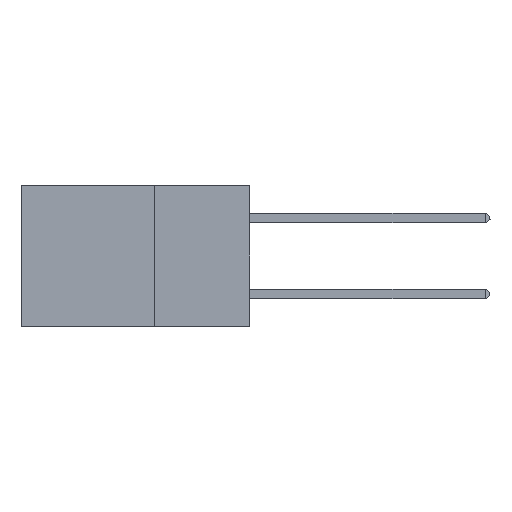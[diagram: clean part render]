
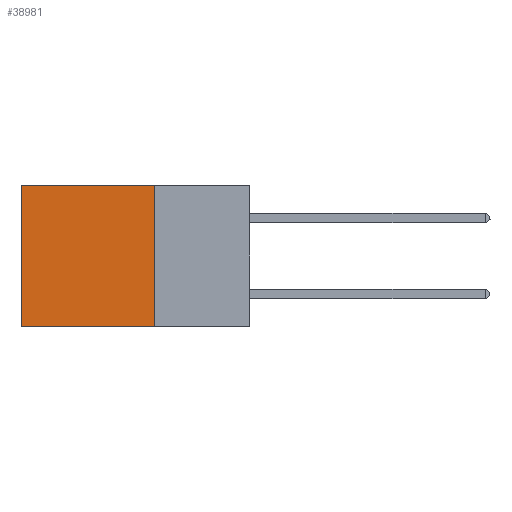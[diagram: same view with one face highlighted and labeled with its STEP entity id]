
A CAD part, left-side view. The second image highlights one B-rep face of the part: STEP entity #38981.
In plain terms, the highlighted planar face has unit normal (-1, 0, 0).
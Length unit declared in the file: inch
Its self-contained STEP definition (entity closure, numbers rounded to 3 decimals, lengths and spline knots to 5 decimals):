
#586 = CARTESIAN_POINT ( 'NONE',  ( 0.2875, 0.6, -0.37 ) ) ;
#1732 = ORIENTED_EDGE ( 'NONE', *, *, #22450, .T. ) ;
#2287 = DIRECTION ( 'NONE',  ( 0., 0., -1. ) ) ;
#5880 = ORIENTED_EDGE ( 'NONE', *, *, #6147, .F. ) ;
#6147 = EDGE_CURVE ( 'NONE', #39737, #12681, #35643, .T. ) ;
#6818 = CARTESIAN_POINT ( 'NONE',  ( 0.2875, 0.25, 0. ) ) ;
#7216 = DIRECTION ( 'NONE',  ( 0., 1., 0. ) ) ;
#8172 = LINE ( 'NONE', #26784, #22308 ) ;
#8890 = CARTESIAN_POINT ( 'NONE',  ( 0.2875, 0.6, 0. ) ) ;
#9580 = EDGE_CURVE ( 'NONE', #12681, #25426, #8172, .T. ) ;
#10699 = LINE ( 'NONE', #23042, #35092 ) ;
#10723 = FACE_OUTER_BOUND ( 'NONE', #15365, .T. ) ;
#11767 = VECTOR ( 'NONE', #7216, 39.37008 ) ;
#12681 = VERTEX_POINT ( 'NONE', #36235 ) ;
#15365 = EDGE_LOOP ( 'NONE', ( #1732, #17955, #5880, #24210 ) ) ;
#17170 = DIRECTION ( 'NONE',  ( 0., 0., -1. ) ) ;
#17955 = ORIENTED_EDGE ( 'NONE', *, *, #9580, .F. ) ;
#19360 = LINE ( 'NONE', #29624, #11767 ) ;
#20217 = EDGE_CURVE ( 'NONE', #39737, #22034, #19360, .T. ) ;
#21104 = DIRECTION ( 'NONE',  ( 0., 1., 0. ) ) ;
#22034 = VERTEX_POINT ( 'NONE', #8890 ) ;
#22308 = VECTOR ( 'NONE', #21104, 39.37008 ) ;
#22450 = EDGE_CURVE ( 'NONE', #22034, #25426, #10699, .T. ) ;
#23042 = CARTESIAN_POINT ( 'NONE',  ( 0.2875, 0.6, 0. ) ) ;
#23856 = AXIS2_PLACEMENT_3D ( 'NONE', #25895, #38225, #26092 ) ;
#24210 = ORIENTED_EDGE ( 'NONE', *, *, #20217, .T. ) ;
#25426 = VERTEX_POINT ( 'NONE', #586 ) ;
#25895 = CARTESIAN_POINT ( 'NONE',  ( 0.2875, 0.25, 0. ) ) ;
#26092 = DIRECTION ( 'NONE',  ( 0., 0., -1. ) ) ;
#26784 = CARTESIAN_POINT ( 'NONE',  ( 0.2875, 0.25, -0.37 ) ) ;
#29568 = CARTESIAN_POINT ( 'NONE',  ( 0.2875, 0.25, 0. ) ) ;
#29624 = CARTESIAN_POINT ( 'NONE',  ( 0.2875, 0.25, 0. ) ) ;
#35092 = VECTOR ( 'NONE', #17170, 39.37008 ) ;
#35643 = LINE ( 'NONE', #29568, #39585 ) ;
#36235 = CARTESIAN_POINT ( 'NONE',  ( 0.2875, 0.25, -0.37 ) ) ;
#38225 = DIRECTION ( 'NONE',  ( 1., 0., 0. ) ) ;
#38428 = PLANE ( 'NONE',  #23856 ) ;
#38981 = ADVANCED_FACE ( 'NONE', ( #10723 ), #38428, .F. ) ;
#39585 = VECTOR ( 'NONE', #2287, 39.37008 ) ;
#39737 = VERTEX_POINT ( 'NONE', #6818 ) ;
